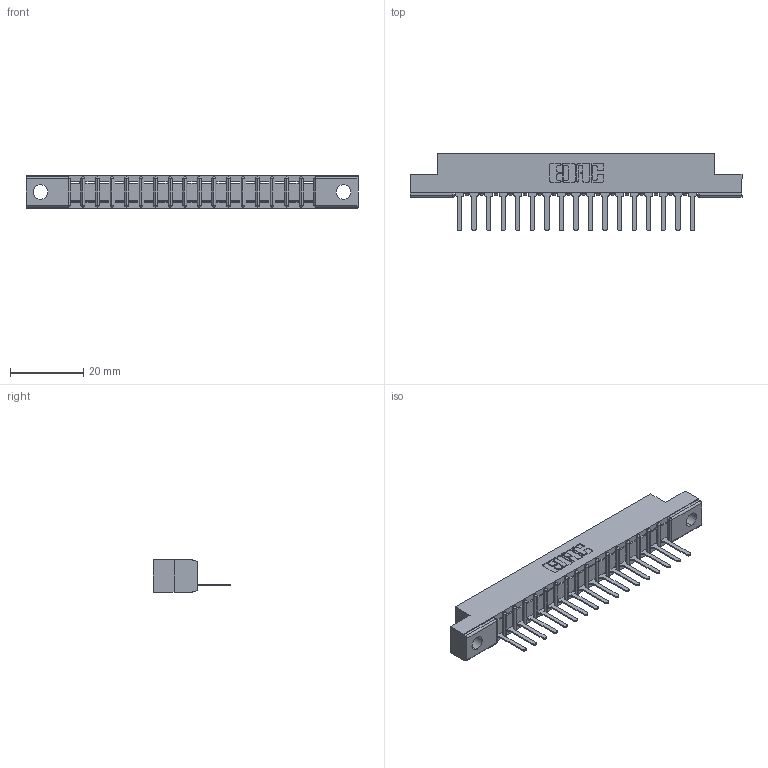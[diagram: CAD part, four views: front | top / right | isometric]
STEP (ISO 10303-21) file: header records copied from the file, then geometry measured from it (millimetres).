
FILE_DESCRIPTION (( 'STEP AP203' ), '1' );
FILE_NAME ('307-017-527-104.STEP', '2019-09-03T17:30:08', ( '' ), ( '' ), 'SwSTEP 2.0', 'SolidWorks 2016', '' );
FILE_SCHEMA (( 'CONFIG_CONTROL_DESIGN' ));
Length unit declared in the file: inch
Products named in the file (3): 307-017-527-104; 307 Part_.156 Dia Mounting Holes; 307-290-001_527
Assembly tree (18 placements, depth 2):
  307-017-527-104
    307 Part_.156 Dia Mounting Holes
    307-290-001_527  x17
Bounding box: 90.37 x 21.11 x 8.71 mm (x, y, z)
Volume: 5623.3 mm3; surface area: 8456.7 mm2
Topology: 18 solids, 18 shells, 1102 faces, 3113 edges, 2002 vertices
Faces by surface type: plane 713, cylinder 353, sphere 36
Entity records: 18042 total; most frequent: CARTESIAN_POINT 3034, ORIENTED_EDGE 3018, DIRECTION 2957, EDGE_CURVE 1509, LINE 1155, VECTOR 1155, VERTEX_POINT 978, AXIS2_PLACEMENT_3D 901
